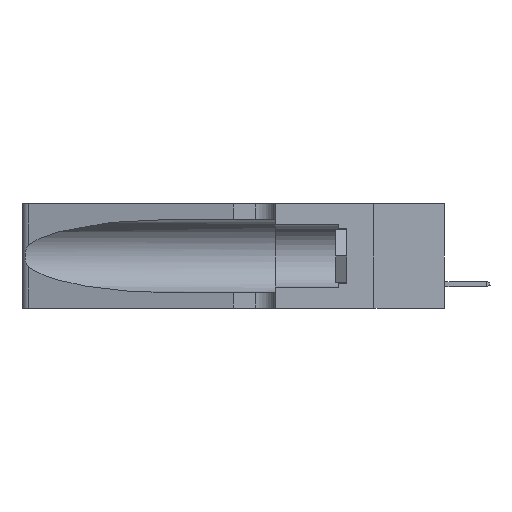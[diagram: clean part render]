
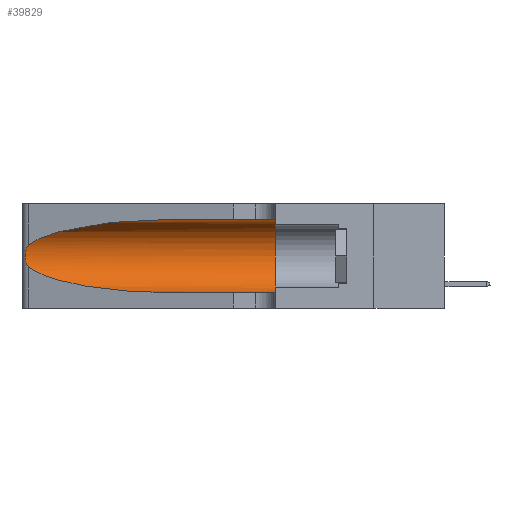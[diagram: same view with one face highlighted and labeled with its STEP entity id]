
A CAD part, left-side view. The second image highlights one B-rep face of the part: STEP entity #39829.
In plain terms, the highlighted cylindrical face has radius 3.308 mm (diameter 6.617 mm), a partial arc.
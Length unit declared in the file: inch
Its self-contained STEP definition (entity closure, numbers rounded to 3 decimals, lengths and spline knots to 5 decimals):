
#1879 = CARTESIAN_POINT ( 'NONE',  ( 0.2373, 1.15595, 0.28018 ) ) ;
#1901 = DIRECTION ( 'NONE',  ( 0., 1., 0. ) ) ;
#1934 = VERTEX_POINT ( 'NONE', #19733 ) ;
#2578 = ORIENTED_EDGE ( 'NONE', *, *, #24391, .T. ) ;
#3525 = FACE_OUTER_BOUND ( 'NONE', #33291, .T. ) ;
#4376 = CARTESIAN_POINT ( 'NONE',  ( 0.1305, 1.61858, 0.185 ) ) ;
#5115 = CYLINDRICAL_SURFACE ( 'NONE', #13520, 0.13025 ) ;
#6533 = CARTESIAN_POINT ( 'NONE',  ( 0.25639, 1.23184, 0.21858 ) ) ;
#6985 = ORIENTED_EDGE ( 'NONE', *, *, #25002, .T. ) ;
#7485 = CARTESIAN_POINT ( 'NONE',  ( 0.18966, 0.96281, 0.31525 ) ) ;
#7689 =( BOUNDED_CURVE ( )  B_SPLINE_CURVE ( 3, ( #28808, #42281, #25508, #42437 ),
 .UNSPECIFIED., .F., .T. ) 
 B_SPLINE_CURVE_WITH_KNOTS ( ( 4, 4 ),
 ( 3.44316, 4.71239 ),
 .UNSPECIFIED. ) 
 CURVE ( )  GEOMETRIC_REPRESENTATION_ITEM ( )  RATIONAL_B_SPLINE_CURVE ( ( 1., 0.87, 0.87, 1. ) ) 
 REPRESENTATION_ITEM ( '' )  );
#8471 = CARTESIAN_POINT ( 'NONE',  ( 0.25487, 1.22718, 0.22369 ) ) ;
#8988 = VERTEX_POINT ( 'NONE', #28853 ) ;
#9000 = CARTESIAN_POINT ( 'NONE',  ( 0.25487, 1.22718, 0.14631 ) ) ;
#10225 =( BOUNDED_CURVE ( )  B_SPLINE_CURVE ( 3, ( #42379, #7485, #1879, #25602 ),
 .UNSPECIFIED., .F., .T. ) 
 B_SPLINE_CURVE_WITH_KNOTS ( ( 4, 4 ),
 ( 1.5708, 2.84003 ),
 .UNSPECIFIED. ) 
 CURVE ( )  GEOMETRIC_REPRESENTATION_ITEM ( )  RATIONAL_B_SPLINE_CURVE ( ( 1., 0.87, 0.87, 1. ) ) 
 REPRESENTATION_ITEM ( '' )  );
#10349 = CARTESIAN_POINT ( 'NONE',  ( 0.25787, 1.23484, 0.2124 ) ) ;
#12271 = VERTEX_POINT ( 'NONE', #16490 ) ;
#13520 = AXIS2_PLACEMENT_3D ( 'NONE', #4376, #31820, #34882 ) ;
#14644 = CARTESIAN_POINT ( 'NONE',  ( 0.25487, 1.22718, 0.22369 ) ) ;
#14872 = CARTESIAN_POINT ( 'NONE',  ( 0.1305, 1.61858, 0.05475 ) ) ;
#15219 = LINE ( 'NONE', #14872, #23175 ) ;
#15464 = VERTEX_POINT ( 'NONE', #9000 ) ;
#15507 = VERTEX_POINT ( 'NONE', #32870 ) ;
#15632 = B_SPLINE_CURVE_WITH_KNOTS ( 'NONE', 3,
 ( #14644, #16996, #6533, #10349, #40343, #23934, #37390, #23519, #24638, #37649, #23330, #19247, #27483, #25565 ),
 .UNSPECIFIED., .F., .F.,
 ( 4, 2, 2, 2, 2, 2, 4 ),
 ( 0., 0.00027, 0.00053, 0.00107, 0.0016, 0.00187, 0.00214 ),
 .UNSPECIFIED. ) ;
#16227 = ORIENTED_EDGE ( 'NONE', *, *, #20248, .T. ) ;
#16490 = CARTESIAN_POINT ( 'NONE',  ( 0.1305, 0.35, 0.31525 ) ) ;
#16996 = CARTESIAN_POINT ( 'NONE',  ( 0.25555, 1.22994, 0.2215 ) ) ;
#17537 = ORIENTED_EDGE ( 'NONE', *, *, #28339, .F. ) ;
#18978 = DIRECTION ( 'NONE',  ( 0., 0., 1. ) ) ;
#19247 = CARTESIAN_POINT ( 'NONE',  ( 0.25639, 1.23186, 0.15144 ) ) ;
#19732 = AXIS2_PLACEMENT_3D ( 'NONE', #42408, #1901, #18978 ) ;
#19733 = CARTESIAN_POINT ( 'NONE',  ( 0.1305, 0.35, 0.05475 ) ) ;
#20248 = EDGE_CURVE ( 'NONE', #25016, #15464, #15632, .T. ) ;
#23175 = VECTOR ( 'NONE', #37888, 39.37008 ) ;
#23330 = CARTESIAN_POINT ( 'NONE',  ( 0.25789, 1.23486, 0.15765 ) ) ;
#23519 = CARTESIAN_POINT ( 'NONE',  ( 0.26075, 1.23896, 0.178 ) ) ;
#23737 = DIRECTION ( 'NONE',  ( 0., -1., 0. ) ) ;
#23934 = CARTESIAN_POINT ( 'NONE',  ( 0.26018, 1.23835, 0.19895 ) ) ;
#24391 = EDGE_CURVE ( 'NONE', #15507, #1934, #15219, .T. ) ;
#24638 = CARTESIAN_POINT ( 'NONE',  ( 0.26017, 1.23833, 0.17102 ) ) ;
#25002 = EDGE_CURVE ( 'NONE', #15464, #15507, #7689, .T. ) ;
#25016 = VERTEX_POINT ( 'NONE', #8471 ) ;
#25508 = CARTESIAN_POINT ( 'NONE',  ( 0.18966, 0.96281, 0.05475 ) ) ;
#25565 = CARTESIAN_POINT ( 'NONE',  ( 0.25487, 1.22718, 0.14631 ) ) ;
#25602 = CARTESIAN_POINT ( 'NONE',  ( 0.25487, 1.22718, 0.22369 ) ) ;
#26455 = VECTOR ( 'NONE', #23737, 39.37008 ) ;
#27483 = CARTESIAN_POINT ( 'NONE',  ( 0.25555, 1.22993, 0.14849 ) ) ;
#28000 = LINE ( 'NONE', #36364, #26455 ) ;
#28339 = EDGE_CURVE ( 'NONE', #12271, #1934, #37103, .T. ) ;
#28808 = CARTESIAN_POINT ( 'NONE',  ( 0.25487, 1.22718, 0.14631 ) ) ;
#28853 = CARTESIAN_POINT ( 'NONE',  ( 0.1305, 0.72297, 0.31525 ) ) ;
#29273 = ORIENTED_EDGE ( 'NONE', *, *, #29680, .F. ) ;
#29680 = EDGE_CURVE ( 'NONE', #8988, #12271, #28000, .T. ) ;
#31820 = DIRECTION ( 'NONE',  ( 0., -1., 0. ) ) ;
#32070 = EDGE_CURVE ( 'NONE', #8988, #25016, #10225, .T. ) ;
#32870 = CARTESIAN_POINT ( 'NONE',  ( 0.1305, 0.72297, 0.05475 ) ) ;
#33291 = EDGE_LOOP ( 'NONE', ( #41770, #16227, #6985, #2578, #17537, #29273 ) ) ;
#34882 = DIRECTION ( 'NONE',  ( 0., 0., -1. ) ) ;
#36364 = CARTESIAN_POINT ( 'NONE',  ( 0.1305, 1.61858, 0.31525 ) ) ;
#37103 = CIRCLE ( 'NONE', #19732, 0.13025 ) ;
#37390 = CARTESIAN_POINT ( 'NONE',  ( 0.26075, 1.23896, 0.19203 ) ) ;
#37649 = CARTESIAN_POINT ( 'NONE',  ( 0.25856, 1.23593, 0.16098 ) ) ;
#37888 = DIRECTION ( 'NONE',  ( 0., -1., 0. ) ) ;
#39829 = ADVANCED_FACE ( 'NONE', ( #3525 ), #5115, .F. ) ;
#40343 = CARTESIAN_POINT ( 'NONE',  ( 0.25854, 1.2359, 0.20912 ) ) ;
#41770 = ORIENTED_EDGE ( 'NONE', *, *, #32070, .T. ) ;
#42281 = CARTESIAN_POINT ( 'NONE',  ( 0.2373, 1.15595, 0.08982 ) ) ;
#42379 = CARTESIAN_POINT ( 'NONE',  ( 0.1305, 0.72297, 0.31525 ) ) ;
#42408 = CARTESIAN_POINT ( 'NONE',  ( 0.1305, 0.35, 0.185 ) ) ;
#42437 = CARTESIAN_POINT ( 'NONE',  ( 0.1305, 0.72297, 0.05475 ) ) ;
